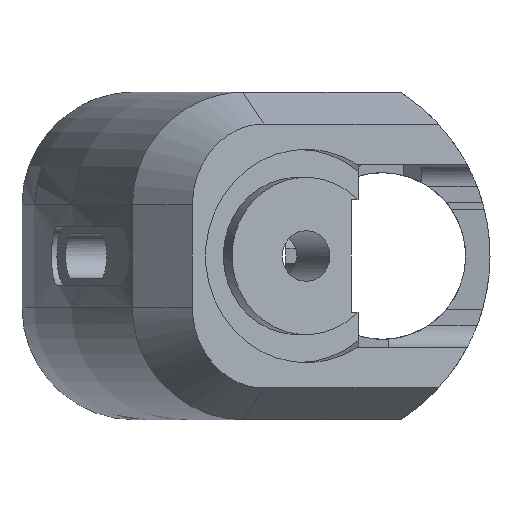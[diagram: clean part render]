
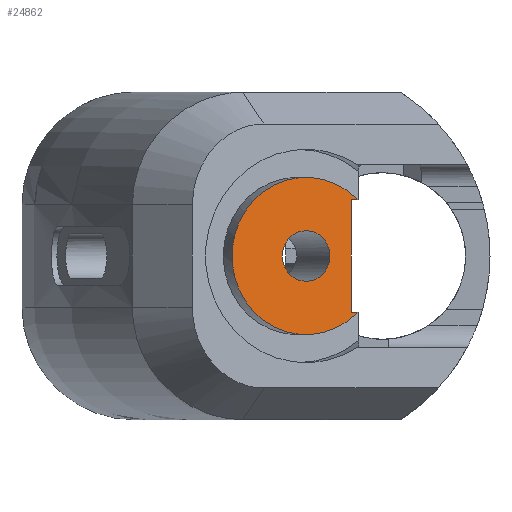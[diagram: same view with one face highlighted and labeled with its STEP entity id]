
A CAD part, left-side view. The second image highlights one B-rep face of the part: STEP entity #24862.
In plain terms, the highlighted planar face has unit normal (-0.943, -0.334, 0).
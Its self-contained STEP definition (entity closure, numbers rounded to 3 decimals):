
#21125 = PLANE('',#21126);
#21126 = AXIS2_PLACEMENT_3D('',#21127,#21128,#21129);
#21127 = CARTESIAN_POINT('',(-152.4,18.796,7.62));
#21128 = DIRECTION('',(0.,-1.,0.));
#21129 = DIRECTION('',(0.,0.,-1.));
#21174 = CYLINDRICAL_SURFACE('',#21175,3.429);
#21175 = AXIS2_PLACEMENT_3D('',#21176,#21177,#21178);
#21176 = CARTESIAN_POINT('',(-202.64,24.947,
    0.));
#21177 = DIRECTION('',(-0.943,-0.334,
    0.));
#21178 = DIRECTION('',(0.334,-0.943,0.
    ));
#21325 = CYLINDRICAL_SURFACE('',#21326,10.668);
#21326 = AXIS2_PLACEMENT_3D('',#21327,#21328,#21329);
#21327 = CARTESIAN_POINT('',(-202.64,24.947,
    0.));
#21328 = DIRECTION('',(-0.943,-0.334,
    0.));
#21329 = DIRECTION('',(0.334,-0.943,0.)
  );
#22631 = VERTEX_POINT('',#22632);
#22632 = CARTESIAN_POINT('',(-200.461,18.796,7.62));
#22646 = PLANE('',#22647);
#22647 = AXIS2_PLACEMENT_3D('',#22648,#22649,#22650);
#22648 = CARTESIAN_POINT('',(-152.4,17.78,7.62));
#22649 = DIRECTION('',(0.,0.,-1.));
#22650 = DIRECTION('',(0.,1.,0.));
#22658 = EDGE_CURVE('',#22631,#22659,#22661,.T.);
#22659 = VERTEX_POINT('',#22660);
#22660 = CARTESIAN_POINT('',(-200.461,18.796,-7.62));
#22661 = SURFACE_CURVE('',#22662,(#22666,#22672),.PCURVE_S1.);
#22662 = LINE('',#22663,#22664);
#22663 = CARTESIAN_POINT('',(-200.461,18.796,-7.303));
#22664 = VECTOR('',#22665,1.);
#22665 = DIRECTION('',(0.,0.,-1.));
#22666 = PCURVE('',#21125,#22667);
#22667 = DEFINITIONAL_REPRESENTATION('',(#22668),#22671);
#22668 = B_SPLINE_CURVE_WITH_KNOTS('',1,(#22669,#22670),.UNSPECIFIED.,
  .F.,.F.,(2,2),(-14.923,0.318),.PIECEWISE_BEZIER_KNOTS.);
#22669 = CARTESIAN_POINT('',(0.,-48.061));
#22670 = CARTESIAN_POINT('',(15.24,-48.061));
#22671 = ( GEOMETRIC_REPRESENTATION_CONTEXT(2) 
PARAMETRIC_REPRESENTATION_CONTEXT() REPRESENTATION_CONTEXT('2D SPACE',''
  ) );
#22672 = PCURVE('',#22673,#22678);
#22673 = PLANE('',#22674);
#22674 = AXIS2_PLACEMENT_3D('',#22675,#22676,#22677);
#22675 = CARTESIAN_POINT('',(-209.55,44.45,-22.225));
#22676 = DIRECTION('',(0.943,0.334,0.
    ));
#22677 = DIRECTION('',(0.334,-0.943,0.
    ));
#22678 = DEFINITIONAL_REPRESENTATION('',(#22679),#22682);
#22679 = B_SPLINE_CURVE_WITH_KNOTS('',1,(#22680,#22681),.UNSPECIFIED.,
  .F.,.F.,(2,2),(-14.923,0.318),.PIECEWISE_BEZIER_KNOTS.);
#22680 = CARTESIAN_POINT('',(27.216,-29.845));
#22681 = CARTESIAN_POINT('',(27.216,-14.605));
#22682 = ( GEOMETRIC_REPRESENTATION_CONTEXT(2) 
PARAMETRIC_REPRESENTATION_CONTEXT() REPRESENTATION_CONTEXT('2D SPACE',''
  ) );
#22700 = PLANE('',#22701);
#22701 = AXIS2_PLACEMENT_3D('',#22702,#22703,#22704);
#22702 = CARTESIAN_POINT('',(-152.4,18.796,-7.62));
#22703 = DIRECTION('',(0.,0.,1.));
#22704 = DIRECTION('',(0.,-1.,0.));
#22742 = EDGE_CURVE('',#22743,#22743,#22745,.T.);
#22743 = VERTEX_POINT('',#22744);
#22744 = CARTESIAN_POINT('',(-201.495,21.715,
    0.));
#22745 = SURFACE_CURVE('',#22746,(#22751,#22758),.PCURVE_S1.);
#22746 = CIRCLE('',#22747,3.429);
#22747 = AXIS2_PLACEMENT_3D('',#22748,#22749,#22750);
#22748 = CARTESIAN_POINT('',(-202.64,24.947,
    0.));
#22749 = DIRECTION('',(-0.943,-0.334,
    0.));
#22750 = DIRECTION('',(0.334,-0.943,0.
    ));
#22751 = PCURVE('',#21174,#22752);
#22752 = DEFINITIONAL_REPRESENTATION('',(#22753),#22757);
#22753 = LINE('',#22754,#22755);
#22754 = CARTESIAN_POINT('',(0.,0.));
#22755 = VECTOR('',#22756,1.);
#22756 = DIRECTION('',(1.,0.));
#22757 = ( GEOMETRIC_REPRESENTATION_CONTEXT(2) 
PARAMETRIC_REPRESENTATION_CONTEXT() REPRESENTATION_CONTEXT('2D SPACE',''
  ) );
#22758 = PCURVE('',#22673,#22759);
#22759 = DEFINITIONAL_REPRESENTATION('',(#22760),#22768);
#22760 = ( BOUNDED_CURVE() B_SPLINE_CURVE(2,(#22761,#22762,#22763,#22764
    ,#22765,#22766,#22767),.UNSPECIFIED.,.T.,.F.) 
B_SPLINE_CURVE_WITH_KNOTS((1,2,2,2,2,1),(-2.094,0.,
    2.094,4.189,6.283,8.378),
.UNSPECIFIED.) CURVE() GEOMETRIC_REPRESENTATION_ITEM() 
RATIONAL_B_SPLINE_CURVE((1.,0.5,1.,0.5,1.,0.5,1.)) REPRESENTATION_ITEM(
  '') );
#22761 = CARTESIAN_POINT('',(24.12,-22.225));
#22762 = CARTESIAN_POINT('',(24.12,-28.164));
#22763 = CARTESIAN_POINT('',(18.976,-25.195));
#22764 = CARTESIAN_POINT('',(13.833,-22.225));
#22765 = CARTESIAN_POINT('',(18.976,-19.255));
#22766 = CARTESIAN_POINT('',(24.12,-16.286));
#22767 = CARTESIAN_POINT('',(24.12,-22.225));
#22768 = ( GEOMETRIC_REPRESENTATION_CONTEXT(2) 
PARAMETRIC_REPRESENTATION_CONTEXT() REPRESENTATION_CONTEXT('2D SPACE',''
  ) );
#22796 = EDGE_CURVE('',#22797,#22799,#22801,.T.);
#22797 = VERTEX_POINT('',#22798);
#22798 = CARTESIAN_POINT('',(-200.147,17.91,7.62));
#22799 = VERTEX_POINT('',#22800);
#22800 = CARTESIAN_POINT('',(-200.147,17.91,-7.62));
#22801 = SURFACE_CURVE('',#22802,(#22807,#22814),.PCURVE_S1.);
#22802 = CIRCLE('',#22803,10.668);
#22803 = AXIS2_PLACEMENT_3D('',#22804,#22805,#22806);
#22804 = CARTESIAN_POINT('',(-202.64,24.947,
    0.));
#22805 = DIRECTION('',(-0.943,-0.334,
    0.));
#22806 = DIRECTION('',(0.334,-0.943,0.)
  );
#22807 = PCURVE('',#21325,#22808);
#22808 = DEFINITIONAL_REPRESENTATION('',(#22809),#22813);
#22809 = LINE('',#22810,#22811);
#22810 = CARTESIAN_POINT('',(0.,0.));
#22811 = VECTOR('',#22812,1.);
#22812 = DIRECTION('',(1.,0.));
#22813 = ( GEOMETRIC_REPRESENTATION_CONTEXT(2) 
PARAMETRIC_REPRESENTATION_CONTEXT() REPRESENTATION_CONTEXT('2D SPACE',''
  ) );
#22814 = PCURVE('',#22673,#22815);
#22815 = DEFINITIONAL_REPRESENTATION('',(#22816),#22824);
#22816 = ( BOUNDED_CURVE() B_SPLINE_CURVE(2,(#22817,#22818,#22819,#22820
    ,#22821,#22822,#22823),.UNSPECIFIED.,.T.,.F.) 
B_SPLINE_CURVE_WITH_KNOTS((1,2,2,2,2,1),(-2.094,0.,
    2.094,4.189,6.283,8.378),
.UNSPECIFIED.) CURVE() GEOMETRIC_REPRESENTATION_ITEM() 
RATIONAL_B_SPLINE_CURVE((1.,0.5,1.,0.5,1.,0.5,1.)) REPRESENTATION_ITEM(
  '') );
#22817 = CARTESIAN_POINT('',(31.359,-22.225));
#22818 = CARTESIAN_POINT('',(31.359,-40.703));
#22819 = CARTESIAN_POINT('',(15.357,-31.464));
#22820 = CARTESIAN_POINT('',(-0.645,-22.225));
#22821 = CARTESIAN_POINT('',(15.357,-12.986));
#22822 = CARTESIAN_POINT('',(31.359,-3.747));
#22823 = CARTESIAN_POINT('',(31.359,-22.225));
#22824 = ( GEOMETRIC_REPRESENTATION_CONTEXT(2) 
PARAMETRIC_REPRESENTATION_CONTEXT() REPRESENTATION_CONTEXT('2D SPACE',''
  ) );
#24844 = EDGE_CURVE('',#22659,#22799,#24845,.T.);
#24845 = SURFACE_CURVE('',#24846,(#24850,#24856),.PCURVE_S1.);
#24846 = LINE('',#24847,#24848);
#24847 = CARTESIAN_POINT('',(-202.326,24.059,-7.62));
#24848 = VECTOR('',#24849,1.);
#24849 = DIRECTION('',(0.334,-0.943,0.
    ));
#24850 = PCURVE('',#22700,#24851);
#24851 = DEFINITIONAL_REPRESENTATION('',(#24852),#24855);
#24852 = B_SPLINE_CURVE_WITH_KNOTS('',1,(#24853,#24854),.UNSPECIFIED.,
  .F.,.F.,(2,2),(5.583,6.661),
  .PIECEWISE_BEZIER_KNOTS.);
#24853 = CARTESIAN_POINT('',(0.,-48.061));
#24854 = CARTESIAN_POINT('',(1.016,-47.701));
#24855 = ( GEOMETRIC_REPRESENTATION_CONTEXT(2) 
PARAMETRIC_REPRESENTATION_CONTEXT() REPRESENTATION_CONTEXT('2D SPACE',''
  ) );
#24856 = PCURVE('',#22673,#24857);
#24857 = DEFINITIONAL_REPRESENTATION('',(#24858),#24861);
#24858 = B_SPLINE_CURVE_WITH_KNOTS('',1,(#24859,#24860),.UNSPECIFIED.,
  .F.,.F.,(2,2),(5.583,6.661),
  .PIECEWISE_BEZIER_KNOTS.);
#24859 = CARTESIAN_POINT('',(27.216,-14.605));
#24860 = CARTESIAN_POINT('',(28.294,-14.605));
#24861 = ( GEOMETRIC_REPRESENTATION_CONTEXT(2) 
PARAMETRIC_REPRESENTATION_CONTEXT() REPRESENTATION_CONTEXT('2D SPACE',''
  ) );
#24862 = ADVANCED_FACE('',(#24863,#24887),#22673,.F.);
#24863 = FACE_BOUND('',#24864,.F.);
#24864 = EDGE_LOOP('',(#24865,#24866,#24867,#24886));
#24865 = ORIENTED_EDGE('',*,*,#24844,.T.);
#24866 = ORIENTED_EDGE('',*,*,#22796,.F.);
#24867 = ORIENTED_EDGE('',*,*,#24868,.T.);
#24868 = EDGE_CURVE('',#22797,#22631,#24869,.T.);
#24869 = SURFACE_CURVE('',#24870,(#24874,#24880),.PCURVE_S1.);
#24870 = LINE('',#24871,#24872);
#24871 = CARTESIAN_POINT('',(-202.166,23.607,7.62));
#24872 = VECTOR('',#24873,1.);
#24873 = DIRECTION('',(-0.334,0.943,
    0.));
#24874 = PCURVE('',#22673,#24875);
#24875 = DEFINITIONAL_REPRESENTATION('',(#24876),#24879);
#24876 = B_SPLINE_CURVE_WITH_KNOTS('',1,(#24877,#24878),.UNSPECIFIED.,
  .F.,.F.,(2,2),(-6.182,-5.104),
  .PIECEWISE_BEZIER_KNOTS.);
#24877 = CARTESIAN_POINT('',(28.294,-29.845));
#24878 = CARTESIAN_POINT('',(27.216,-29.845));
#24879 = ( GEOMETRIC_REPRESENTATION_CONTEXT(2) 
PARAMETRIC_REPRESENTATION_CONTEXT() REPRESENTATION_CONTEXT('2D SPACE',''
  ) );
#24880 = PCURVE('',#22646,#24881);
#24881 = DEFINITIONAL_REPRESENTATION('',(#24882),#24885);
#24882 = B_SPLINE_CURVE_WITH_KNOTS('',1,(#24883,#24884),.UNSPECIFIED.,
  .F.,.F.,(2,2),(-6.182,-5.104),
  .PIECEWISE_BEZIER_KNOTS.);
#24883 = CARTESIAN_POINT('',(0.,-47.701));
#24884 = CARTESIAN_POINT('',(1.016,-48.061));
#24885 = ( GEOMETRIC_REPRESENTATION_CONTEXT(2) 
PARAMETRIC_REPRESENTATION_CONTEXT() REPRESENTATION_CONTEXT('2D SPACE',''
  ) );
#24886 = ORIENTED_EDGE('',*,*,#22658,.T.);
#24887 = FACE_BOUND('',#24888,.F.);
#24888 = EDGE_LOOP('',(#24889));
#24889 = ORIENTED_EDGE('',*,*,#22742,.T.);
